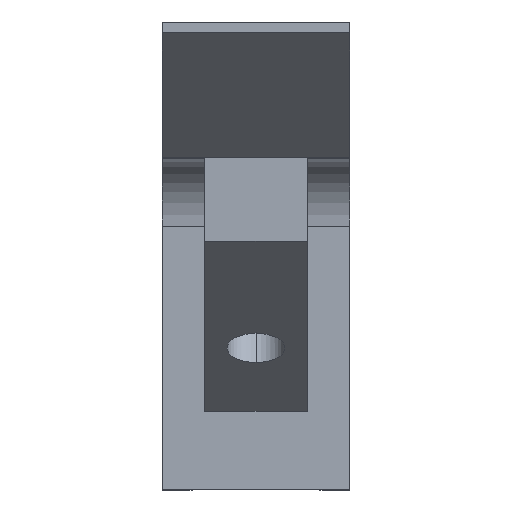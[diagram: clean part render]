
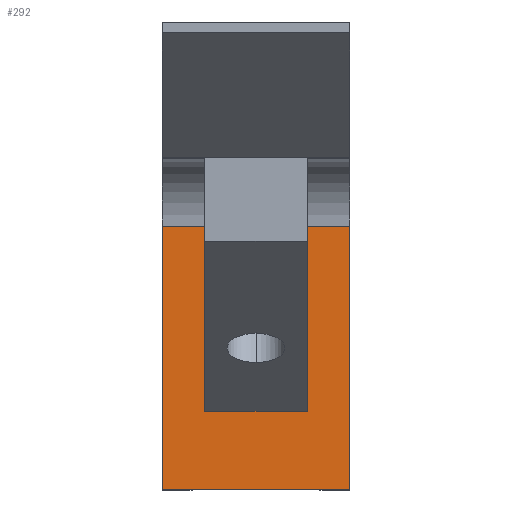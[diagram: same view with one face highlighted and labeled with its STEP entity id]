
A CAD part, top view. The second image highlights one B-rep face of the part: STEP entity #292.
In plain terms, the highlighted planar face has unit normal (0, 0, 1).
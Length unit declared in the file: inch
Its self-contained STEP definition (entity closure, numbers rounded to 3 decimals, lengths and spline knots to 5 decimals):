
#26 = VECTOR ( 'NONE', #454, 39.37008 ) ;
#40 = AXIS2_PLACEMENT_3D ( 'NONE', #848, #1226, #461 ) ;
#48 = EDGE_CURVE ( 'NONE', #386, #1464, #764, .T. ) ;
#52 = EDGE_LOOP ( 'NONE', ( #482, #356, #1354, #1104, #1306, #939, #584, #533 ) ) ;
#79 = VERTEX_POINT ( 'NONE', #555 ) ;
#111 = VECTOR ( 'NONE', #1398, 39.37008 ) ;
#115 = CARTESIAN_POINT ( 'NONE',  ( 0.345, 0., 0.4 ) ) ;
#127 = EDGE_CURVE ( 'NONE', #79, #1464, #1018, .T. ) ;
#184 = LINE ( 'NONE', #1401, #111 ) ;
#250 = CARTESIAN_POINT ( 'NONE',  ( 0.1875, 0.288, 0.4 ) ) ;
#292 = ADVANCED_FACE ( 'NONE', ( #1505 ), #719, .T. ) ;
#309 = DIRECTION ( 'NONE',  ( 0., 1., 0. ) ) ;
#356 = ORIENTED_EDGE ( 'NONE', *, *, #897, .F. ) ;
#381 = DIRECTION ( 'NONE',  ( 0., 1., 0. ) ) ;
#386 = VERTEX_POINT ( 'NONE', #867 ) ;
#412 = CARTESIAN_POINT ( 'NONE',  ( 0.1875, 0.96774, 0.4 ) ) ;
#423 = EDGE_CURVE ( 'NONE', #847, #386, #973, .T. ) ;
#439 = CARTESIAN_POINT ( 'NONE',  ( 0.345, 0., 0.4 ) ) ;
#454 = DIRECTION ( 'NONE',  ( -1., 0., 0. ) ) ;
#461 = DIRECTION ( 'NONE',  ( 1., 0., 0. ) ) ;
#482 = ORIENTED_EDGE ( 'NONE', *, *, #127, .F. ) ;
#533 = ORIENTED_EDGE ( 'NONE', *, *, #48, .T. ) ;
#547 = CARTESIAN_POINT ( 'NONE',  ( -0.1875, 0.288, 0.4 ) ) ;
#555 = CARTESIAN_POINT ( 'NONE',  ( -0.345, 0., 0.4 ) ) ;
#584 = ORIENTED_EDGE ( 'NONE', *, *, #423, .T. ) ;
#619 = CARTESIAN_POINT ( 'NONE',  ( 0.345, 0.96774, 0.4 ) ) ;
#629 = VERTEX_POINT ( 'NONE', #115 ) ;
#669 = LINE ( 'NONE', #412, #1299 ) ;
#681 = DIRECTION ( 'NONE',  ( 0., 1., 0. ) ) ;
#692 = EDGE_CURVE ( 'NONE', #711, #1281, #908, .T. ) ;
#711 = VERTEX_POINT ( 'NONE', #1525 ) ;
#719 = PLANE ( 'NONE',  #40 ) ;
#734 = VECTOR ( 'NONE', #309, 39.37008 ) ;
#764 = LINE ( 'NONE', #842, #26 ) ;
#782 = EDGE_CURVE ( 'NONE', #711, #847, #184, .T. ) ;
#842 = CARTESIAN_POINT ( 'NONE',  ( -0.1875, 0.96774, 0.4 ) ) ;
#847 = VERTEX_POINT ( 'NONE', #547 ) ;
#848 = CARTESIAN_POINT ( 'NONE',  ( 0.345, 0., 0.4 ) ) ;
#867 = CARTESIAN_POINT ( 'NONE',  ( -0.1875, 0.96774, 0.4 ) ) ;
#869 = EDGE_CURVE ( 'NONE', #1281, #1138, #669, .T. ) ;
#897 = EDGE_CURVE ( 'NONE', #629, #79, #1646, .T. ) ;
#908 = LINE ( 'NONE', #250, #1535 ) ;
#939 = ORIENTED_EDGE ( 'NONE', *, *, #782, .T. ) ;
#948 = EDGE_CURVE ( 'NONE', #629, #1138, #1062, .T. ) ;
#973 = LINE ( 'NONE', #1125, #1049 ) ;
#976 = VECTOR ( 'NONE', #681, 39.37008 ) ;
#1018 = LINE ( 'NONE', #1307, #976 ) ;
#1049 = VECTOR ( 'NONE', #1376, 39.37008 ) ;
#1062 = LINE ( 'NONE', #439, #734 ) ;
#1064 = DIRECTION ( 'NONE',  ( 1., 0., 0. ) ) ;
#1104 = ORIENTED_EDGE ( 'NONE', *, *, #869, .F. ) ;
#1125 = CARTESIAN_POINT ( 'NONE',  ( -0.1875, 0.288, 0.4 ) ) ;
#1138 = VERTEX_POINT ( 'NONE', #619 ) ;
#1190 = CARTESIAN_POINT ( 'NONE',  ( 0.345, 0., 0.4 ) ) ;
#1226 = DIRECTION ( 'NONE',  ( 0., 0., 1. ) ) ;
#1281 = VERTEX_POINT ( 'NONE', #1315 ) ;
#1299 = VECTOR ( 'NONE', #1064, 39.37008 ) ;
#1306 = ORIENTED_EDGE ( 'NONE', *, *, #692, .F. ) ;
#1307 = CARTESIAN_POINT ( 'NONE',  ( -0.345, 0., 0.4 ) ) ;
#1315 = CARTESIAN_POINT ( 'NONE',  ( 0.1875, 0.96774, 0.4 ) ) ;
#1354 = ORIENTED_EDGE ( 'NONE', *, *, #948, .T. ) ;
#1376 = DIRECTION ( 'NONE',  ( 0., 1., 0. ) ) ;
#1398 = DIRECTION ( 'NONE',  ( -1., 0., 0. ) ) ;
#1401 = CARTESIAN_POINT ( 'NONE',  ( 0.345, 0.288, 0.4 ) ) ;
#1464 = VERTEX_POINT ( 'NONE', #1495 ) ;
#1495 = CARTESIAN_POINT ( 'NONE',  ( -0.345, 0.96774, 0.4 ) ) ;
#1505 = FACE_OUTER_BOUND ( 'NONE', #52, .T. ) ;
#1525 = CARTESIAN_POINT ( 'NONE',  ( 0.1875, 0.288, 0.4 ) ) ;
#1535 = VECTOR ( 'NONE', #381, 39.37008 ) ;
#1565 = DIRECTION ( 'NONE',  ( -1., 0., 0. ) ) ;
#1600 = VECTOR ( 'NONE', #1565, 39.37008 ) ;
#1646 = LINE ( 'NONE', #1190, #1600 ) ;
